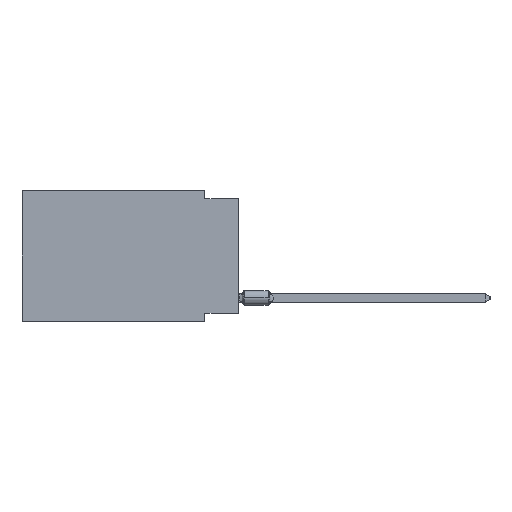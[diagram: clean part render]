
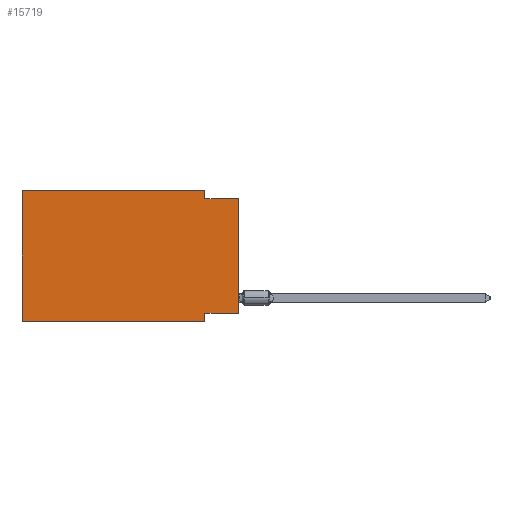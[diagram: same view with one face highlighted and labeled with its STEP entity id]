
A CAD part, left-side view. The second image highlights one B-rep face of the part: STEP entity #15719.
In plain terms, the highlighted planar face has unit normal (-1, 0, 0).
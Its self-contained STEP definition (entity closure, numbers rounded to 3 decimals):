
#280 = VECTOR ( 'NONE', #15903, 1000. ) ;
#519 = DIRECTION ( 'NONE',  ( 0., -1., 0. ) ) ;
#861 = DIRECTION ( 'NONE',  ( 0., 1., 0. ) ) ;
#871 = VECTOR ( 'NONE', #9065, 1000. ) ;
#1432 = AXIS2_PLACEMENT_3D ( 'NONE', #24025, #17791, #35857 ) ;
#1890 = ORIENTED_EDGE ( 'NONE', *, *, #12613, .F. ) ;
#2060 = CARTESIAN_POINT ( 'NONE',  ( 0., 2.54, -0.635 ) ) ;
#2118 = CARTESIAN_POINT ( 'NONE',  ( 0., 0., -0.635 ) ) ;
#2590 = CARTESIAN_POINT ( 'NONE',  ( 0., 16.383, 0. ) ) ;
#4335 = CARTESIAN_POINT ( 'NONE',  ( 0., 0., -0.635 ) ) ;
#5600 = CARTESIAN_POINT ( 'NONE',  ( 0., 2.54, 0. ) ) ;
#5714 = DIRECTION ( 'NONE',  ( 0., 0., 1. ) ) ;
#5972 = PLANE ( 'NONE',  #1432 ) ;
#6285 = ORIENTED_EDGE ( 'NONE', *, *, #41063, .F. ) ;
#6510 = VECTOR ( 'NONE', #8298, 1000. ) ;
#6953 = VERTEX_POINT ( 'NONE', #16663 ) ;
#6986 = ORIENTED_EDGE ( 'NONE', *, *, #40556, .F. ) ;
#8180 = VECTOR ( 'NONE', #519, 1000. ) ;
#8298 = DIRECTION ( 'NONE',  ( 0., 0., 1. ) ) ;
#8520 = EDGE_CURVE ( 'NONE', #6953, #12895, #18991, .T. ) ;
#9065 = DIRECTION ( 'NONE',  ( 0., 0., -1. ) ) ;
#9810 = ORIENTED_EDGE ( 'NONE', *, *, #38896, .T. ) ;
#11265 = ORIENTED_EDGE ( 'NONE', *, *, #8520, .F. ) ;
#12080 = LINE ( 'NONE', #33977, #29171 ) ;
#12093 = CARTESIAN_POINT ( 'NONE',  ( 0., 16.383, 0. ) ) ;
#12613 = EDGE_CURVE ( 'NONE', #34415, #15109, #13081, .T. ) ;
#12895 = VERTEX_POINT ( 'NONE', #36844 ) ;
#13081 = LINE ( 'NONE', #42543, #871 ) ;
#13990 = DIRECTION ( 'NONE',  ( 0., -1., 0. ) ) ;
#15109 = VERTEX_POINT ( 'NONE', #39847 ) ;
#15709 = EDGE_CURVE ( 'NONE', #12895, #44264, #20668, .T. ) ;
#15719 = ADVANCED_FACE ( 'NONE', ( #42531 ), #5972, .F. ) ;
#15903 = DIRECTION ( 'NONE',  ( 0., 0., -1. ) ) ;
#16663 = CARTESIAN_POINT ( 'NONE',  ( 0., 16.383, -9.906 ) ) ;
#17208 = ORIENTED_EDGE ( 'NONE', *, *, #15709, .F. ) ;
#17791 = DIRECTION ( 'NONE',  ( 1., 0., 0. ) ) ;
#18850 = CARTESIAN_POINT ( 'NONE',  ( 0., 2.54, -9.271 ) ) ;
#18991 = LINE ( 'NONE', #12093, #6510 ) ;
#20668 = LINE ( 'NONE', #2590, #38654 ) ;
#23305 = LINE ( 'NONE', #30906, #32341 ) ;
#24025 = CARTESIAN_POINT ( 'NONE',  ( 0., 16.383, 0. ) ) ;
#25528 = VERTEX_POINT ( 'NONE', #2060 ) ;
#26198 = LINE ( 'NONE', #4335, #28342 ) ;
#26627 = ORIENTED_EDGE ( 'NONE', *, *, #30234, .T. ) ;
#26648 = EDGE_CURVE ( 'NONE', #36689, #34415, #12080, .T. ) ;
#28342 = VECTOR ( 'NONE', #44018, 1000. ) ;
#29171 = VECTOR ( 'NONE', #861, 1000. ) ;
#29324 = LINE ( 'NONE', #44502, #8180 ) ;
#29743 = ORIENTED_EDGE ( 'NONE', *, *, #26648, .F. ) ;
#30234 = EDGE_CURVE ( 'NONE', #6953, #15109, #29324, .T. ) ;
#30906 = CARTESIAN_POINT ( 'NONE',  ( 0., 0., 0. ) ) ;
#32341 = VECTOR ( 'NONE', #5714, 1000. ) ;
#33977 = CARTESIAN_POINT ( 'NONE',  ( 0., 0., -9.271 ) ) ;
#34004 = CARTESIAN_POINT ( 'NONE',  ( 0., 2.54, 0. ) ) ;
#34415 = VERTEX_POINT ( 'NONE', #18850 ) ;
#34454 = LINE ( 'NONE', #34004, #280 ) ;
#35857 = DIRECTION ( 'NONE',  ( 0., 0., -1. ) ) ;
#36689 = VERTEX_POINT ( 'NONE', #41324 ) ;
#36844 = CARTESIAN_POINT ( 'NONE',  ( 0., 16.383, 0. ) ) ;
#38654 = VECTOR ( 'NONE', #13990, 1000. ) ;
#38857 = VERTEX_POINT ( 'NONE', #2118 ) ;
#38896 = EDGE_CURVE ( 'NONE', #36689, #38857, #23305, .T. ) ;
#39847 = CARTESIAN_POINT ( 'NONE',  ( 0., 2.54, -9.906 ) ) ;
#40556 = EDGE_CURVE ( 'NONE', #25528, #38857, #26198, .T. ) ;
#41063 = EDGE_CURVE ( 'NONE', #44264, #25528, #34454, .T. ) ;
#41324 = CARTESIAN_POINT ( 'NONE',  ( 0., 0., -9.271 ) ) ;
#42531 = FACE_OUTER_BOUND ( 'NONE', #46467, .T. ) ;
#42543 = CARTESIAN_POINT ( 'NONE',  ( 0., 2.54, -9.906 ) ) ;
#44018 = DIRECTION ( 'NONE',  ( 0., -1., 0. ) ) ;
#44264 = VERTEX_POINT ( 'NONE', #5600 ) ;
#44502 = CARTESIAN_POINT ( 'NONE',  ( 0., 16.383, -9.906 ) ) ;
#46467 = EDGE_LOOP ( 'NONE', ( #9810, #6986, #6285, #17208, #11265, #26627, #1890, #29743 ) ) ;
